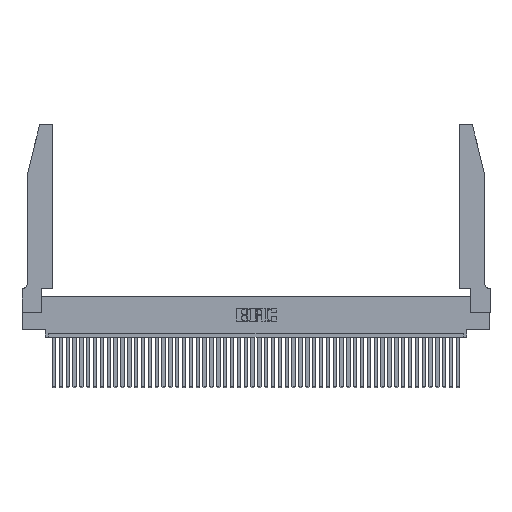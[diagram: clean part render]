
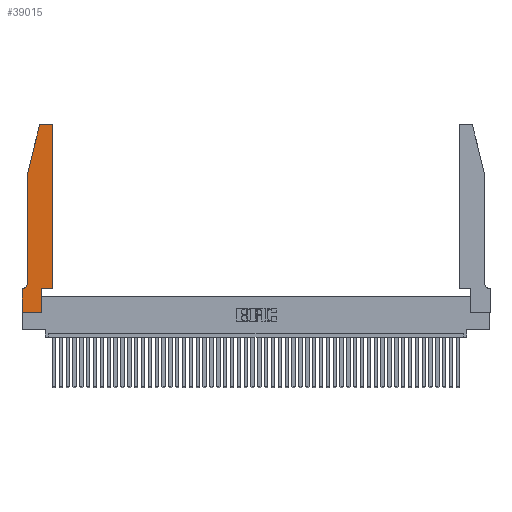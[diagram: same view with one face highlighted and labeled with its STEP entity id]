
A CAD part, top view. The second image highlights one B-rep face of the part: STEP entity #39015.
In plain terms, the highlighted planar face has unit normal (0, 0, 1).
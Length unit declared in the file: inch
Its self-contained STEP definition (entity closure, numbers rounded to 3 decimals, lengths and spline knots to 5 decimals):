
#838 = EDGE_CURVE ( 'NONE', #46164, #31595, #25943, .T. ) ;
#1756 = DIRECTION ( 'NONE',  ( 0., 1., 0. ) ) ;
#1804 = FACE_OUTER_BOUND ( 'NONE', #18104, .T. ) ;
#2014 = EDGE_CURVE ( 'NONE', #2677, #20914, #16672, .T. ) ;
#2328 = ORIENTED_EDGE ( 'NONE', *, *, #838, .T. ) ;
#2525 = CIRCLE ( 'NONE', #34471, 0.07 ) ;
#2677 = VERTEX_POINT ( 'NONE', #29420 ) ;
#3414 = DIRECTION ( 'NONE',  ( -1., 0., 0. ) ) ;
#3969 = ORIENTED_EDGE ( 'NONE', *, *, #26768, .T. ) ;
#4163 = DIRECTION ( 'NONE',  ( 0., 0., -1. ) ) ;
#4259 = LINE ( 'NONE', #43596, #23138 ) ;
#4911 = CARTESIAN_POINT ( 'NONE',  ( 0.25487, 2.72718, 0.37 ) ) ;
#5127 = LINE ( 'NONE', #5935, #14756 ) ;
#5602 = DIRECTION ( 'NONE',  ( 0., -1., 0. ) ) ;
#5935 = CARTESIAN_POINT ( 'NONE',  ( 0.4505, 0.35, 0.37 ) ) ;
#6410 = CARTESIAN_POINT ( 'NONE',  ( 0., 0., 0.37 ) ) ;
#6575 = DIRECTION ( 'NONE',  ( -1., 0., 0. ) ) ;
#6939 = VECTOR ( 'NONE', #38698, 39.37008 ) ;
#7187 = DIRECTION ( 'NONE',  ( 1., 0., 0. ) ) ;
#7754 = LINE ( 'NONE', #6410, #10614 ) ;
#8936 = ORIENTED_EDGE ( 'NONE', *, *, #11161, .T. ) ;
#9399 = CARTESIAN_POINT ( 'NONE',  ( 0., 0., 0.37 ) ) ;
#9870 = CARTESIAN_POINT ( 'NONE',  ( 0.0755, 2., 0.37 ) ) ;
#9939 = EDGE_CURVE ( 'NONE', #15981, #38760, #18890, .T. ) ;
#10200 = ORIENTED_EDGE ( 'NONE', *, *, #16276, .T. ) ;
#10547 = EDGE_CURVE ( 'NONE', #20914, #30447, #32641, .T. ) ;
#10614 = VECTOR ( 'NONE', #20749, 39.37008 ) ;
#11161 = EDGE_CURVE ( 'NONE', #21026, #44769, #5127, .T. ) ;
#12893 = CARTESIAN_POINT ( 'NONE',  ( 0.2865, 0.35, 0.37 ) ) ;
#13115 = CARTESIAN_POINT ( 'NONE',  ( 0., 0.35, 0.37 ) ) ;
#14654 = CARTESIAN_POINT ( 'NONE',  ( 0.4205, 2.75, 0.37 ) ) ;
#14702 = ORIENTED_EDGE ( 'NONE', *, *, #32505, .T. ) ;
#14756 = VECTOR ( 'NONE', #7187, 39.37008 ) ;
#14891 = EDGE_CURVE ( 'NONE', #38760, #2677, #17945, .T. ) ;
#15372 = DIRECTION ( 'NONE',  ( 0., 1., 0. ) ) ;
#15981 = VERTEX_POINT ( 'NONE', #18765 ) ;
#16276 = EDGE_CURVE ( 'NONE', #20061, #21026, #24996, .T. ) ;
#16672 = CIRCLE ( 'NONE', #24901, 0.03 ) ;
#16776 = VECTOR ( 'NONE', #15372, 39.37008 ) ;
#16880 = DIRECTION ( 'NONE',  ( 0., 0., 1. ) ) ;
#17945 = LINE ( 'NONE', #28451, #37939 ) ;
#18104 = EDGE_LOOP ( 'NONE', ( #23268, #29912, #43863, #34645, #24957, #14702, #2328, #3969, #10200, #8936, #29132, #22689 ) ) ;
#18208 = CARTESIAN_POINT ( 'NONE',  ( 0.4505, 0.35, 0.37 ) ) ;
#18765 = CARTESIAN_POINT ( 'NONE',  ( 0.4505, 2.72, 0.37 ) ) ;
#18890 = CIRCLE ( 'NONE', #25080, 0.03 ) ;
#19158 = CARTESIAN_POINT ( 'NONE',  ( 0.0755, 2., 0.37 ) ) ;
#19644 = VECTOR ( 'NONE', #5602, 39.37008 ) ;
#20061 = VERTEX_POINT ( 'NONE', #24265 ) ;
#20740 = CARTESIAN_POINT ( 'NONE',  ( 0.4205, 2.72, 0.37 ) ) ;
#20749 = DIRECTION ( 'NONE',  ( 1., 0., 0. ) ) ;
#20914 = VERTEX_POINT ( 'NONE', #4911 ) ;
#20942 = AXIS2_PLACEMENT_3D ( 'NONE', #13115, #39240, #24170 ) ;
#21026 = VERTEX_POINT ( 'NONE', #37299 ) ;
#21192 = CARTESIAN_POINT ( 'NONE',  ( 0.0055, 0.35, 0.37 ) ) ;
#22386 = CARTESIAN_POINT ( 'NONE',  ( 0., 0.35, 0.37 ) ) ;
#22689 = ORIENTED_EDGE ( 'NONE', *, *, #9939, .T. ) ;
#23138 = VECTOR ( 'NONE', #3414, 39.37008 ) ;
#23268 = ORIENTED_EDGE ( 'NONE', *, *, #14891, .T. ) ;
#24170 = DIRECTION ( 'NONE',  ( 1., 0., 0. ) ) ;
#24265 = CARTESIAN_POINT ( 'NONE',  ( 0.2865, 0., 0.37 ) ) ;
#24658 = PLANE ( 'NONE',  #20942 ) ;
#24816 = DIRECTION ( 'NONE',  ( 0., 0., 1. ) ) ;
#24901 = AXIS2_PLACEMENT_3D ( 'NONE', #27500, #24816, #31186 ) ;
#24957 = ORIENTED_EDGE ( 'NONE', *, *, #40673, .T. ) ;
#24996 = LINE ( 'NONE', #12893, #40993 ) ;
#25080 = AXIS2_PLACEMENT_3D ( 'NONE', #20740, #16880, #31651 ) ;
#25943 = LINE ( 'NONE', #45280, #19644 ) ;
#25977 = VERTEX_POINT ( 'NONE', #30437 ) ;
#26071 = CARTESIAN_POINT ( 'NONE',  ( 0.0055, 0.42, 0.37 ) ) ;
#26494 = LINE ( 'NONE', #30116, #16776 ) ;
#26768 = EDGE_CURVE ( 'NONE', #31595, #20061, #7754, .T. ) ;
#27500 = CARTESIAN_POINT ( 'NONE',  ( 0.284, 2.72, 0.37 ) ) ;
#28451 = CARTESIAN_POINT ( 'NONE',  ( 0.2605, 2.75, 0.37 ) ) ;
#29132 = ORIENTED_EDGE ( 'NONE', *, *, #37281, .T. ) ;
#29420 = CARTESIAN_POINT ( 'NONE',  ( 0.284, 2.75, 0.37 ) ) ;
#29912 = ORIENTED_EDGE ( 'NONE', *, *, #2014, .T. ) ;
#30116 = CARTESIAN_POINT ( 'NONE',  ( 0.4505, 0.35, 0.37 ) ) ;
#30437 = CARTESIAN_POINT ( 'NONE',  ( 0.0755, 0.42, 0.37 ) ) ;
#30447 = VERTEX_POINT ( 'NONE', #45012 ) ;
#30468 = VECTOR ( 'NONE', #37608, 39.37008 ) ;
#31186 = DIRECTION ( 'NONE',  ( 1., 0., 0. ) ) ;
#31595 = VERTEX_POINT ( 'NONE', #9399 ) ;
#31651 = DIRECTION ( 'NONE',  ( 1., 0., 0. ) ) ;
#32505 = EDGE_CURVE ( 'NONE', #36440, #46164, #4259, .T. ) ;
#32641 = LINE ( 'NONE', #9870, #6939 ) ;
#34471 = AXIS2_PLACEMENT_3D ( 'NONE', #26071, #4163, #37442 ) ;
#34516 = LINE ( 'NONE', #19158, #30468 ) ;
#34645 = ORIENTED_EDGE ( 'NONE', *, *, #40643, .T. ) ;
#36440 = VERTEX_POINT ( 'NONE', #21192 ) ;
#37281 = EDGE_CURVE ( 'NONE', #44769, #15981, #26494, .T. ) ;
#37299 = CARTESIAN_POINT ( 'NONE',  ( 0.2865, 0.35, 0.37 ) ) ;
#37442 = DIRECTION ( 'NONE',  ( -1., 0., 0. ) ) ;
#37608 = DIRECTION ( 'NONE',  ( 0., -1., 0. ) ) ;
#37939 = VECTOR ( 'NONE', #6575, 39.37008 ) ;
#38698 = DIRECTION ( 'NONE',  ( -0.239, -0.971, 0. ) ) ;
#38760 = VERTEX_POINT ( 'NONE', #14654 ) ;
#39015 = ADVANCED_FACE ( 'NONE', ( #1804 ), #24658, .T. ) ;
#39240 = DIRECTION ( 'NONE',  ( 0., 0., 1. ) ) ;
#40643 = EDGE_CURVE ( 'NONE', #30447, #25977, #34516, .T. ) ;
#40673 = EDGE_CURVE ( 'NONE', #25977, #36440, #2525, .T. ) ;
#40993 = VECTOR ( 'NONE', #1756, 39.37008 ) ;
#43596 = CARTESIAN_POINT ( 'NONE',  ( 0.0755, 0.35, 0.37 ) ) ;
#43863 = ORIENTED_EDGE ( 'NONE', *, *, #10547, .T. ) ;
#44769 = VERTEX_POINT ( 'NONE', #18208 ) ;
#45012 = CARTESIAN_POINT ( 'NONE',  ( 0.0755, 2., 0.37 ) ) ;
#45280 = CARTESIAN_POINT ( 'NONE',  ( 0., 0., 0.37 ) ) ;
#46164 = VERTEX_POINT ( 'NONE', #22386 ) ;
